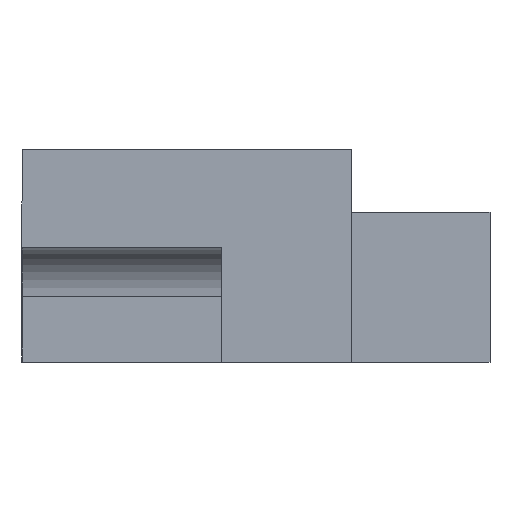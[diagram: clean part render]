
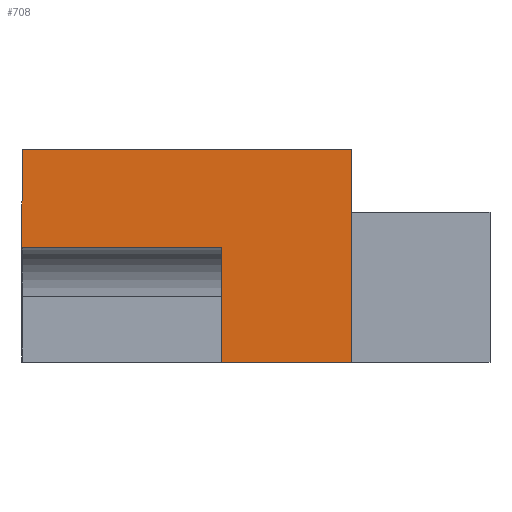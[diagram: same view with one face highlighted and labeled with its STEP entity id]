
A CAD part, left-side view. The second image highlights one B-rep face of the part: STEP entity #708.
In plain terms, the highlighted planar face has unit normal (-1, 0, 0).
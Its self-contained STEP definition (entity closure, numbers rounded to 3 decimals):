
#448 = ORIENTED_EDGE ( 'NONE', *, *, #21694, .F. ) ;
#708 = ADVANCED_FACE ( 'NONE', ( #18793 ), #23936, .F. ) ;
#1630 = CARTESIAN_POINT ( 'NONE',  ( 0., 0., 0. ) ) ;
#2139 = LINE ( 'NONE', #22931, #4654 ) ;
#2239 = ORIENTED_EDGE ( 'NONE', *, *, #20048, .F. ) ;
#2806 = DIRECTION ( 'NONE',  ( 0., 0., 1. ) ) ;
#3312 = DIRECTION ( 'NONE',  ( 0., 0., -1. ) ) ;
#3903 = EDGE_LOOP ( 'NONE', ( #2239, #448, #10094, #11193, #20350, #11577 ) ) ;
#4654 = VECTOR ( 'NONE', #14845, 1000. ) ;
#5081 = CARTESIAN_POINT ( 'NONE',  ( 0., 20.955, -13.487 ) ) ;
#6317 = VERTEX_POINT ( 'NONE', #24896 ) ;
#6596 = CARTESIAN_POINT ( 'NONE',  ( 0., 8.255, -13.487 ) ) ;
#7700 = EDGE_CURVE ( 'NONE', #11487, #24706, #25945, .T. ) ;
#8119 = VECTOR ( 'NONE', #17284, 1000. ) ;
#8536 = CARTESIAN_POINT ( 'NONE',  ( 0., 11.506, 0. ) ) ;
#9165 = VECTOR ( 'NONE', #25281, 1000. ) ;
#9851 = CARTESIAN_POINT ( 'NONE',  ( 0., 0., 0. ) ) ;
#9942 = VERTEX_POINT ( 'NONE', #11323 ) ;
#10094 = ORIENTED_EDGE ( 'NONE', *, *, #13515, .F. ) ;
#10162 = DIRECTION ( 'NONE',  ( 0., 1., 0. ) ) ;
#10661 = LINE ( 'NONE', #17379, #8119 ) ;
#11193 = ORIENTED_EDGE ( 'NONE', *, *, #7700, .F. ) ;
#11323 = CARTESIAN_POINT ( 'NONE',  ( 0., 8.255, -6.172 ) ) ;
#11487 = VERTEX_POINT ( 'NONE', #12814 ) ;
#11577 = ORIENTED_EDGE ( 'NONE', *, *, #19403, .F. ) ;
#12814 = CARTESIAN_POINT ( 'NONE',  ( 0., 20.955, -6.172 ) ) ;
#13020 = AXIS2_PLACEMENT_3D ( 'NONE', #1630, #24017, #3312 ) ;
#13515 = EDGE_CURVE ( 'NONE', #24706, #17203, #18530, .T. ) ;
#13880 = VERTEX_POINT ( 'NONE', #18808 ) ;
#14845 = DIRECTION ( 'NONE',  ( 0., 1., 0. ) ) ;
#17194 = VECTOR ( 'NONE', #23493, 1000. ) ;
#17203 = VERTEX_POINT ( 'NONE', #9851 ) ;
#17249 = LINE ( 'NONE', #18319, #22037 ) ;
#17284 = DIRECTION ( 'NONE',  ( 0., 0., -1. ) ) ;
#17379 = CARTESIAN_POINT ( 'NONE',  ( 0., 0., 0. ) ) ;
#18319 = CARTESIAN_POINT ( 'NONE',  ( 0., 8.255, -6.172 ) ) ;
#18530 = LINE ( 'NONE', #8536, #17194 ) ;
#18793 = FACE_OUTER_BOUND ( 'NONE', #3903, .T. ) ;
#18808 = CARTESIAN_POINT ( 'NONE',  ( 0., 8.255, -13.487 ) ) ;
#19198 = EDGE_CURVE ( 'NONE', #9942, #11487, #17249, .T. ) ;
#19403 = EDGE_CURVE ( 'NONE', #13880, #9942, #21972, .T. ) ;
#20048 = EDGE_CURVE ( 'NONE', #6317, #13880, #2139, .T. ) ;
#20350 = ORIENTED_EDGE ( 'NONE', *, *, #19198, .F. ) ;
#20541 = CARTESIAN_POINT ( 'NONE',  ( 0., 20.955, 0. ) ) ;
#20823 = VECTOR ( 'NONE', #2806, 1000. ) ;
#21694 = EDGE_CURVE ( 'NONE', #17203, #6317, #10661, .T. ) ;
#21972 = LINE ( 'NONE', #6596, #9165 ) ;
#22037 = VECTOR ( 'NONE', #10162, 1000. ) ;
#22931 = CARTESIAN_POINT ( 'NONE',  ( 0., -8.814, -13.487 ) ) ;
#23493 = DIRECTION ( 'NONE',  ( 0., -1., 0. ) ) ;
#23936 = PLANE ( 'NONE',  #13020 ) ;
#24017 = DIRECTION ( 'NONE',  ( 1., 0., 0. ) ) ;
#24706 = VERTEX_POINT ( 'NONE', #20541 ) ;
#24896 = CARTESIAN_POINT ( 'NONE',  ( 0., 0., -13.487 ) ) ;
#25281 = DIRECTION ( 'NONE',  ( 0., 0., 1. ) ) ;
#25945 = LINE ( 'NONE', #5081, #20823 ) ;
